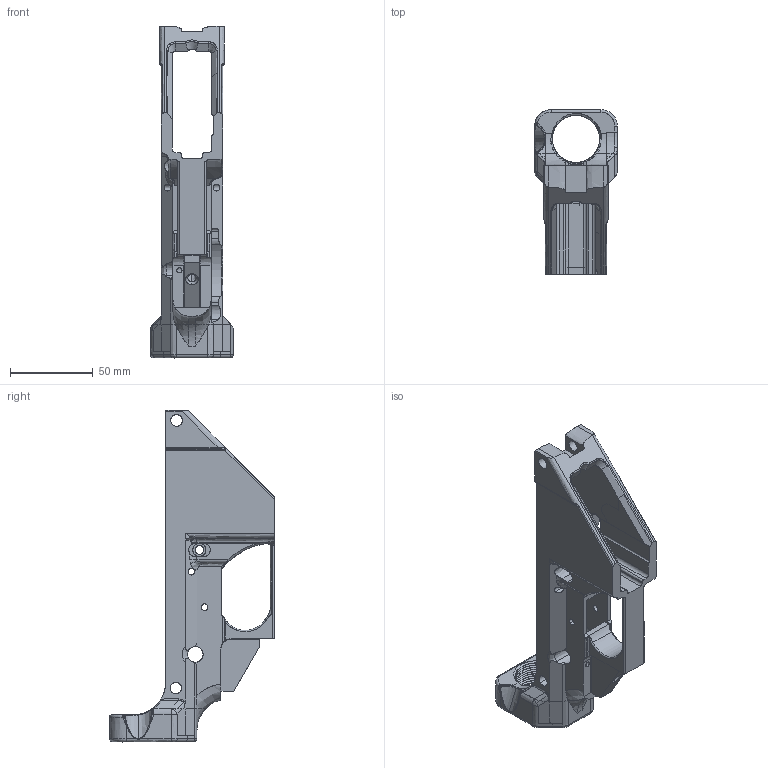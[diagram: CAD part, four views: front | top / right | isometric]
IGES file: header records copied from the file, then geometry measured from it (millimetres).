
Start section: SolidWorks IGES file using analytic representation for surfaces
Global section: file name: JT_Vanguard_Update FP.IGS; native system: SolidWorks 2015; preprocessor: SolidWorks 2015; author: AK0490; date: 150901.182733; units: millimetre
Bounding box: 50 x 99.72 x 200.87 mm (x, y, z)
Surface area: 59205.9 mm2 (no closed solid volume)
Topology: 0 solids, 0 shells, 600 faces, 7901 edges, 7893 vertices
Faces by surface type: bspline 327, revolution 273
